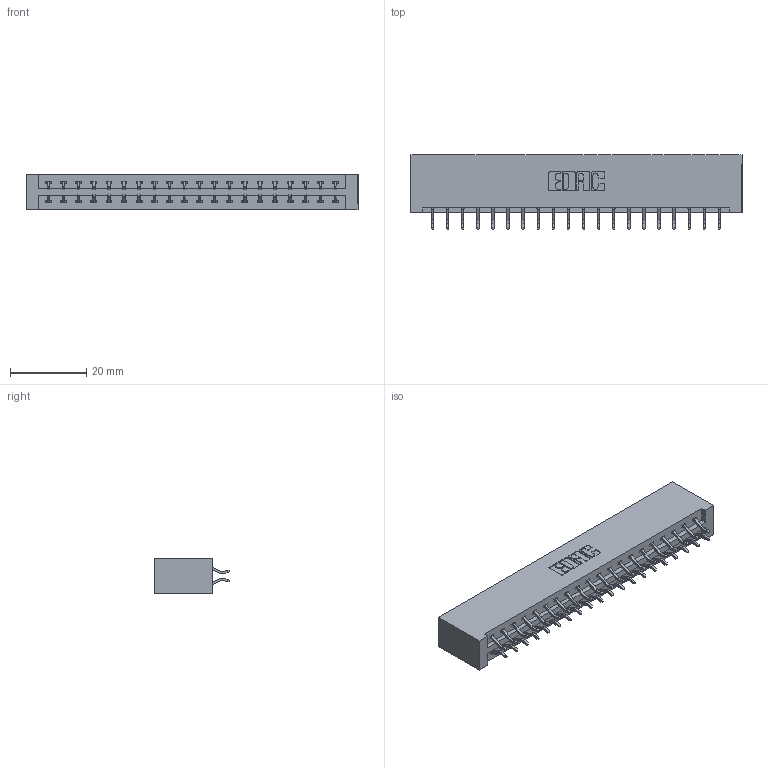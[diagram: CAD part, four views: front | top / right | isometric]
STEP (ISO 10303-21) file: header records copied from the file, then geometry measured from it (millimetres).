
FILE_DESCRIPTION (( 'STEP AP203' ), '1' );
FILE_NAME ('387-040-556-201.STEP', '2018-09-19T16:55:37', ( '' ), ( '' ), 'SwSTEP 2.0', 'SolidWorks 2016', '' );
FILE_SCHEMA (( 'CONFIG_CONTROL_DESIGN' ));
Length unit declared in the file: inch
Products named in the file (3): 337 Part_No Mounting Lugs; 345-292-001_556 Tail; 387-040-556-201
Assembly tree (41 placements, depth 2):
  387-040-556-201
    337 Part_No Mounting Lugs
    345-292-001_556 Tail  x40
Bounding box: 87.12 x 19.57 x 9.4 mm (x, y, z)
Volume: 9647.9 mm3; surface area: 10707.2 mm2
Topology: 41 solids, 41 shells, 2506 faces, 7447 edges, 4910 vertices
Faces by surface type: plane 1746, cylinder 760
Entity records: 18295 total; most frequent: CARTESIAN_POINT 3114, ORIENTED_EDGE 3038, DIRECTION 2671, EDGE_CURVE 1519, VECTOR 1391, LINE 1391, VERTEX_POINT 1010, AXIS2_PLACEMENT_3D 640
